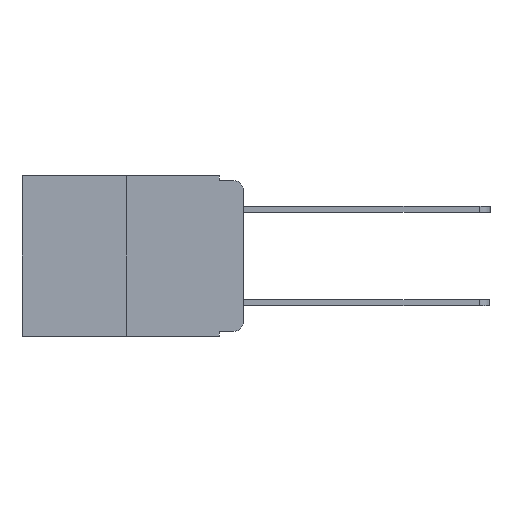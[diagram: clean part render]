
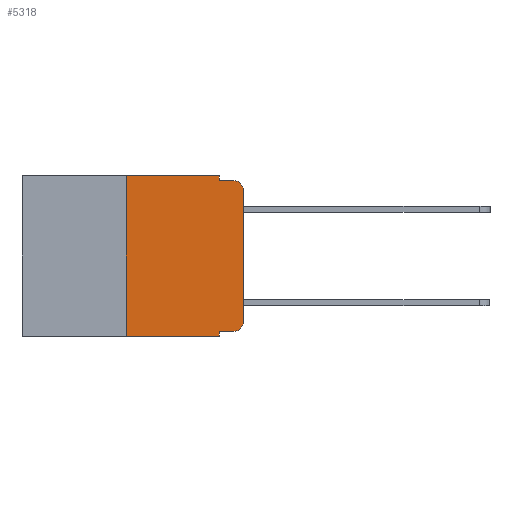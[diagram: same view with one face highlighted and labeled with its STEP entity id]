
A CAD part, left-side view. The second image highlights one B-rep face of the part: STEP entity #5318.
In plain terms, the highlighted planar face has unit normal (-1, 0, 0).
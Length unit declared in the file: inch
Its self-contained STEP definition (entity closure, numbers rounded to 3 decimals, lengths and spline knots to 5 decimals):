
#299 = ORIENTED_EDGE ( 'NONE', *, *, #11999, .T. ) ;
#342 = CARTESIAN_POINT ( 'NONE',  ( 0., 0.473, 0. ) ) ;
#521 = DIRECTION ( 'NONE',  ( 0., 0., 1. ) ) ;
#532 = VERTEX_POINT ( 'NONE', #12493 ) ;
#749 = VECTOR ( 'NONE', #13700, 39.37008 ) ;
#901 = VECTOR ( 'NONE', #521, 39.37008 ) ;
#995 = LINE ( 'NONE', #7428, #13622 ) ;
#1437 = DIRECTION ( 'NONE',  ( 0., 0., -1. ) ) ;
#1767 = ORIENTED_EDGE ( 'NONE', *, *, #4637, .T. ) ;
#2286 = FACE_OUTER_BOUND ( 'NONE', #20302, .T. ) ;
#2337 = CIRCLE ( 'NONE', #16691, 0.02 ) ;
#2627 = EDGE_CURVE ( 'NONE', #3476, #17662, #3531, .T. ) ;
#2731 = VERTEX_POINT ( 'NONE', #8984 ) ;
#3016 = ORIENTED_EDGE ( 'NONE', *, *, #2627, .F. ) ;
#3050 = VECTOR ( 'NONE', #9032, 39.37008 ) ;
#3476 = VERTEX_POINT ( 'NONE', #11430 ) ;
#3531 = LINE ( 'NONE', #342, #7495 ) ;
#4054 = CARTESIAN_POINT ( 'NONE',  ( 0., 0.02, -0.313 ) ) ;
#4228 = CARTESIAN_POINT ( 'NONE',  ( 0., 0.051, -0.01 ) ) ;
#4271 = VERTEX_POINT ( 'NONE', #13861 ) ;
#4624 = ORIENTED_EDGE ( 'NONE', *, *, #19255, .T. ) ;
#4637 = EDGE_CURVE ( 'NONE', #2731, #20468, #14391, .T. ) ;
#5318 = ADVANCED_FACE ( 'NONE', ( #2286 ), #10613, .F. ) ;
#5838 = DIRECTION ( 'NONE',  ( 0., 0., -1. ) ) ;
#6292 = DIRECTION ( 'NONE',  ( 0., -1., 0. ) ) ;
#6293 = VERTEX_POINT ( 'NONE', #14411 ) ;
#6576 = VERTEX_POINT ( 'NONE', #14353 ) ;
#6948 = VECTOR ( 'NONE', #7002, 39.37008 ) ;
#7002 = DIRECTION ( 'NONE',  ( 0., 0., 1. ) ) ;
#7419 = ORIENTED_EDGE ( 'NONE', *, *, #10981, .T. ) ;
#7428 = CARTESIAN_POINT ( 'NONE',  ( 0., 0.051, -0.333 ) ) ;
#7495 = VECTOR ( 'NONE', #19966, 39.37008 ) ;
#7499 = ORIENTED_EDGE ( 'NONE', *, *, #18234, .T. ) ;
#7982 = CARTESIAN_POINT ( 'NONE',  ( 0., 0.051, 0. ) ) ;
#8064 = DIRECTION ( 'NONE',  ( 0., 0., -1. ) ) ;
#8984 = CARTESIAN_POINT ( 'NONE',  ( 0., 0.25, -0.343 ) ) ;
#9003 = CARTESIAN_POINT ( 'NONE',  ( 0., 0., 0. ) ) ;
#9032 = DIRECTION ( 'NONE',  ( 0., 0., -1. ) ) ;
#9042 = LINE ( 'NONE', #7982, #16860 ) ;
#9449 = VERTEX_POINT ( 'NONE', #4228 ) ;
#9831 = ORIENTED_EDGE ( 'NONE', *, *, #15175, .F. ) ;
#10241 = VECTOR ( 'NONE', #6292, 39.37008 ) ;
#10383 = LINE ( 'NONE', #9003, #901 ) ;
#10437 = CIRCLE ( 'NONE', #15373, 0.02 ) ;
#10613 = PLANE ( 'NONE',  #17772 ) ;
#10981 = EDGE_CURVE ( 'NONE', #4271, #6576, #2337, .T. ) ;
#11430 = CARTESIAN_POINT ( 'NONE',  ( 0., 0.25, 0. ) ) ;
#11436 = DIRECTION ( 'NONE',  ( -1., 0., 0. ) ) ;
#11999 = EDGE_CURVE ( 'NONE', #6293, #4271, #995, .T. ) ;
#12124 = CARTESIAN_POINT ( 'NONE',  ( 0., 0.051, -0.01 ) ) ;
#12493 = CARTESIAN_POINT ( 'NONE',  ( 0., 0., -0.03 ) ) ;
#13542 = CARTESIAN_POINT ( 'NONE',  ( 0., 0.051, -0.343 ) ) ;
#13622 = VECTOR ( 'NONE', #19920, 39.37008 ) ;
#13700 = DIRECTION ( 'NONE',  ( 0., -1., 0. ) ) ;
#13779 = CARTESIAN_POINT ( 'NONE',  ( 0., 0.02, -0.01 ) ) ;
#13861 = CARTESIAN_POINT ( 'NONE',  ( 0., 0.02, -0.333 ) ) ;
#13895 = LINE ( 'NONE', #12124, #749 ) ;
#14109 = EDGE_CURVE ( 'NONE', #6293, #20468, #15509, .T. ) ;
#14353 = CARTESIAN_POINT ( 'NONE',  ( 0., 0., -0.313 ) ) ;
#14391 = LINE ( 'NONE', #17635, #10241 ) ;
#14411 = CARTESIAN_POINT ( 'NONE',  ( 0., 0.051, -0.333 ) ) ;
#14957 = DIRECTION ( 'NONE',  ( 1., 0., 0. ) ) ;
#15175 = EDGE_CURVE ( 'NONE', #2731, #3476, #15438, .T. ) ;
#15189 = ORIENTED_EDGE ( 'NONE', *, *, #17237, .F. ) ;
#15325 = VERTEX_POINT ( 'NONE', #13779 ) ;
#15373 = AXIS2_PLACEMENT_3D ( 'NONE', #20658, #11436, #1437 ) ;
#15390 = DIRECTION ( 'NONE',  ( -1., 0., 0. ) ) ;
#15438 = LINE ( 'NONE', #16500, #6948 ) ;
#15509 = LINE ( 'NONE', #18340, #3050 ) ;
#16188 = EDGE_CURVE ( 'NONE', #17662, #9449, #9042, .T. ) ;
#16279 = CARTESIAN_POINT ( 'NONE',  ( 0., 0.051, 0. ) ) ;
#16500 = CARTESIAN_POINT ( 'NONE',  ( 0., 0.25, 0. ) ) ;
#16691 = AXIS2_PLACEMENT_3D ( 'NONE', #4054, #15390, #5838 ) ;
#16860 = VECTOR ( 'NONE', #8064, 39.37008 ) ;
#17237 = EDGE_CURVE ( 'NONE', #9449, #15325, #13895, .T. ) ;
#17635 = CARTESIAN_POINT ( 'NONE',  ( 0., 0.473, -0.343 ) ) ;
#17662 = VERTEX_POINT ( 'NONE', #16279 ) ;
#17772 = AXIS2_PLACEMENT_3D ( 'NONE', #17946, #14957, #20713 ) ;
#17840 = ORIENTED_EDGE ( 'NONE', *, *, #14109, .F. ) ;
#17946 = CARTESIAN_POINT ( 'NONE',  ( 0., 0.473, 0. ) ) ;
#18234 = EDGE_CURVE ( 'NONE', #532, #15325, #10437, .T. ) ;
#18340 = CARTESIAN_POINT ( 'NONE',  ( 0., 0.051, 0. ) ) ;
#19255 = EDGE_CURVE ( 'NONE', #6576, #532, #10383, .T. ) ;
#19920 = DIRECTION ( 'NONE',  ( 0., -1., 0. ) ) ;
#19966 = DIRECTION ( 'NONE',  ( 0., -1., 0. ) ) ;
#20244 = ORIENTED_EDGE ( 'NONE', *, *, #16188, .F. ) ;
#20302 = EDGE_LOOP ( 'NONE', ( #4624, #7499, #15189, #20244, #3016, #9831, #1767, #17840, #299, #7419 ) ) ;
#20468 = VERTEX_POINT ( 'NONE', #13542 ) ;
#20658 = CARTESIAN_POINT ( 'NONE',  ( 0., 0.02, -0.03 ) ) ;
#20713 = DIRECTION ( 'NONE',  ( 0., 0., -1. ) ) ;
